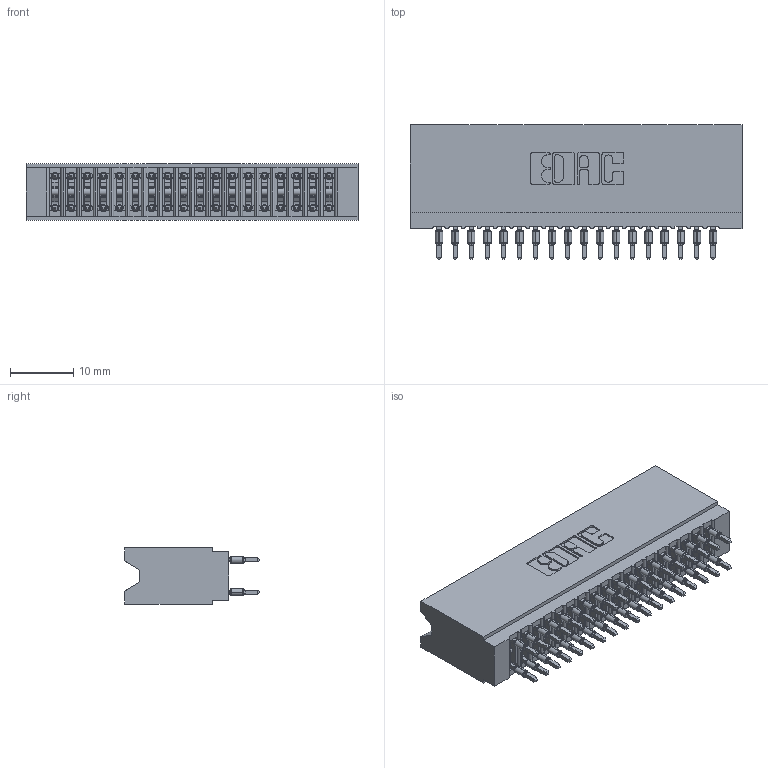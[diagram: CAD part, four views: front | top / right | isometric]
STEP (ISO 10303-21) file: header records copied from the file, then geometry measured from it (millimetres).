
FILE_DESCRIPTION (( 'STEP AP203' ), '1' );
FILE_NAME ('745-036-560-206.STEP', '2026-02-26T17:22:10', ( '' ), ( '' ), 'SwSTEP 2.0', 'SolidWorks 2023', '' );
FILE_SCHEMA (( 'CONFIG_CONTROL_DESIGN' ));
Length unit declared in the file: millimetre
Products named in the file (3): 745-292-001_560; 745 Part_Insulator Option - 06; 745-036-560-206
Assembly tree (37 placements, depth 2):
  745-036-560-206
    745 Part_Insulator Option - 06
    745-292-001_560  x36
Bounding box: 52.32 x 21.22 x 8.89 mm (x, y, z)
Volume: 4967.9 mm3; surface area: 10138.8 mm2
Topology: 37 solids, 37 shells, 3642 faces, 9962 edges, 6328 vertices
Faces by surface type: plane 1892, cylinder 814, bspline 720, torus 216
Entity records: 33923 total; most frequent: CARTESIAN_POINT 6396, ORIENTED_EDGE 5784, DIRECTION 5078, EDGE_CURVE 2892, LINE 2594, VECTOR 2594, VERTEX_POINT 1848, AXIS2_PLACEMENT_3D 1242
